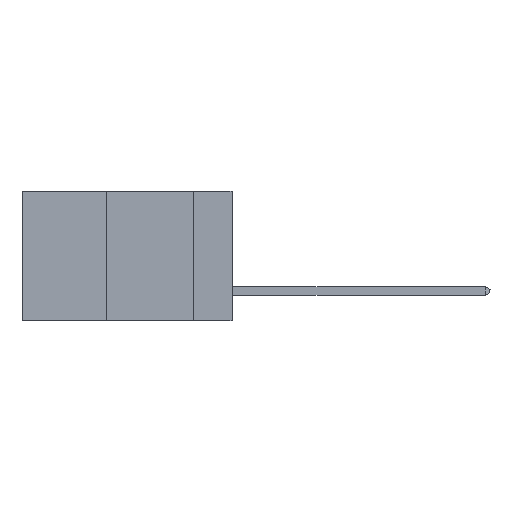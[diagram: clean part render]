
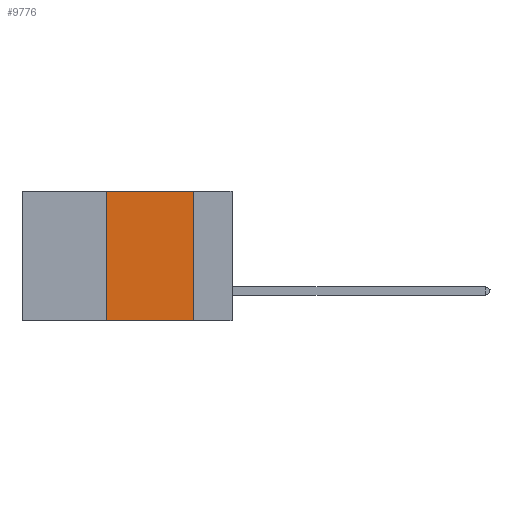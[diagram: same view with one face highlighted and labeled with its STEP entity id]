
A CAD part, left-side view. The second image highlights one B-rep face of the part: STEP entity #9776.
In plain terms, the highlighted planar face has unit normal (-1, 0, 0).
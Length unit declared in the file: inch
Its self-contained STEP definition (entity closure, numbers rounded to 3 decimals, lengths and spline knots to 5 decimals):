
#301 = CARTESIAN_POINT ( 'NONE',  ( 0., 0.11, -0.37 ) ) ;
#438 = DIRECTION ( 'NONE',  ( 0., -1., 0. ) ) ;
#439 = DIRECTION ( 'NONE',  ( 0., 0., 1. ) ) ;
#516 = CARTESIAN_POINT ( 'NONE',  ( 0., 0.11, 0. ) ) ;
#2299 = ORIENTED_EDGE ( 'NONE', *, *, #13564, .F. ) ;
#2597 = EDGE_CURVE ( 'NONE', #11835, #7842, #6581, .T. ) ;
#3164 = FACE_OUTER_BOUND ( 'NONE', #3867, .T. ) ;
#3358 = CARTESIAN_POINT ( 'NONE',  ( 0., 0.6, 0. ) ) ;
#3867 = EDGE_LOOP ( 'NONE', ( #2299, #14221, #6552, #5772 ) ) ;
#4471 = DIRECTION ( 'NONE',  ( 0., 0., -1. ) ) ;
#4968 = LINE ( 'NONE', #11548, #6285 ) ;
#5772 = ORIENTED_EDGE ( 'NONE', *, *, #15288, .T. ) ;
#5823 = CARTESIAN_POINT ( 'NONE',  ( 0., 0.36, 0. ) ) ;
#5917 = VERTEX_POINT ( 'NONE', #516 ) ;
#6285 = VECTOR ( 'NONE', #438, 39.37008 ) ;
#6340 = DIRECTION ( 'NONE',  ( 0., -1., 0. ) ) ;
#6347 = EDGE_CURVE ( 'NONE', #7842, #5917, #9326, .T. ) ;
#6552 = ORIENTED_EDGE ( 'NONE', *, *, #2597, .F. ) ;
#6581 = LINE ( 'NONE', #14912, #12496 ) ;
#6711 = CARTESIAN_POINT ( 'NONE',  ( 0., 0.11, 0. ) ) ;
#7034 = LINE ( 'NONE', #6711, #13372 ) ;
#7194 = VECTOR ( 'NONE', #6340, 39.37008 ) ;
#7842 = VERTEX_POINT ( 'NONE', #5823 ) ;
#8200 = VERTEX_POINT ( 'NONE', #301 ) ;
#8270 = DIRECTION ( 'NONE',  ( 1., 0., 0. ) ) ;
#9326 = LINE ( 'NONE', #11462, #7194 ) ;
#9776 = ADVANCED_FACE ( 'NONE', ( #3164 ), #11904, .F. ) ;
#9864 = CARTESIAN_POINT ( 'NONE',  ( 0., 0.36, -0.37 ) ) ;
#11462 = CARTESIAN_POINT ( 'NONE',  ( 0., 0.6, 0. ) ) ;
#11548 = CARTESIAN_POINT ( 'NONE',  ( 0., 0.6, -0.37 ) ) ;
#11642 = DIRECTION ( 'NONE',  ( 0., 0., -1. ) ) ;
#11835 = VERTEX_POINT ( 'NONE', #9864 ) ;
#11904 = PLANE ( 'NONE',  #12622 ) ;
#12496 = VECTOR ( 'NONE', #439, 39.37008 ) ;
#12622 = AXIS2_PLACEMENT_3D ( 'NONE', #3358, #8270, #4471 ) ;
#13372 = VECTOR ( 'NONE', #11642, 39.37008 ) ;
#13564 = EDGE_CURVE ( 'NONE', #5917, #8200, #7034, .T. ) ;
#14221 = ORIENTED_EDGE ( 'NONE', *, *, #6347, .F. ) ;
#14912 = CARTESIAN_POINT ( 'NONE',  ( 0., 0.36, 0. ) ) ;
#15288 = EDGE_CURVE ( 'NONE', #11835, #8200, #4968, .T. ) ;
